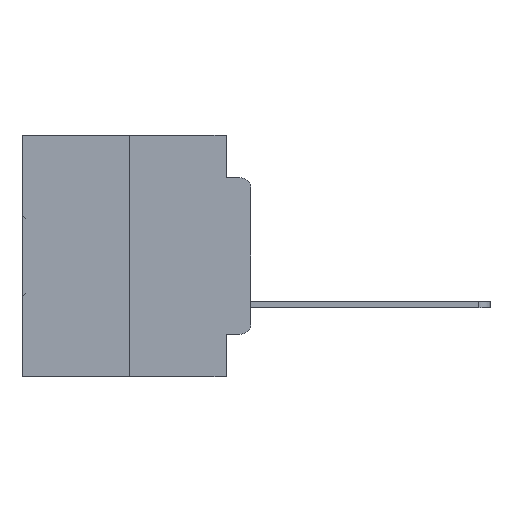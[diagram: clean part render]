
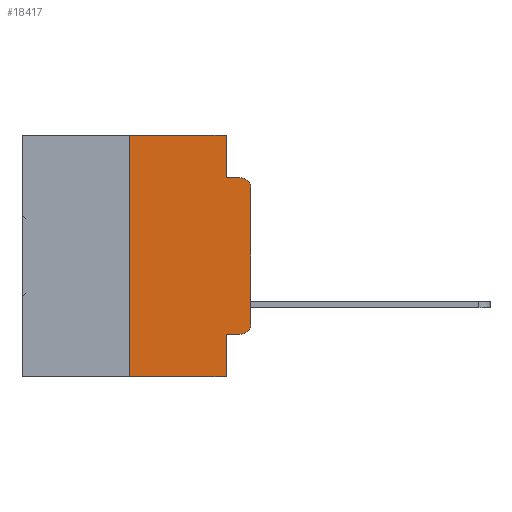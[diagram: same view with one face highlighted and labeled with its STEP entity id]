
A CAD part, left-side view. The second image highlights one B-rep face of the part: STEP entity #18417.
In plain terms, the highlighted planar face has unit normal (-1, 0, 0).
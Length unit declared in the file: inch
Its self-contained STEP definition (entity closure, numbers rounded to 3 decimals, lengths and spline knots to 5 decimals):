
#1 = LINE ( 'NONE', #24178, #26257 ) ;
#377 = VERTEX_POINT ( 'NONE', #13164 ) ;
#1495 = VECTOR ( 'NONE', #8526, 39.37008 ) ;
#1611 = DIRECTION ( 'NONE',  ( 0., -1., 0. ) ) ;
#2806 = DIRECTION ( 'NONE',  ( 0., 0., 1. ) ) ;
#3068 = CARTESIAN_POINT ( 'NONE',  ( 0., 0.051, -0.5 ) ) ;
#4232 = VERTEX_POINT ( 'NONE', #7900 ) ;
#4436 = LINE ( 'NONE', #25506, #17606 ) ;
#4638 = DIRECTION ( 'NONE',  ( -1., 0., 0. ) ) ;
#5345 = CARTESIAN_POINT ( 'NONE',  ( 0., 0.02, -0.4115 ) ) ;
#5774 = CARTESIAN_POINT ( 'NONE',  ( 0., 0.051, -0.0885 ) ) ;
#5888 = CARTESIAN_POINT ( 'NONE',  ( 0., 0.051, 0. ) ) ;
#7290 = LINE ( 'NONE', #23462, #27106 ) ;
#7723 = CARTESIAN_POINT ( 'NONE',  ( 0., 0.473, 0. ) ) ;
#7900 = CARTESIAN_POINT ( 'NONE',  ( 0., 0.051, -0.4115 ) ) ;
#8096 = CARTESIAN_POINT ( 'NONE',  ( 0., 0.25, -0.5 ) ) ;
#8526 = DIRECTION ( 'NONE',  ( 0., 0., -1. ) ) ;
#8541 = VECTOR ( 'NONE', #29583, 39.37008 ) ;
#10542 = AXIS2_PLACEMENT_3D ( 'NONE', #7723, #10728, #28582 ) ;
#10728 = DIRECTION ( 'NONE',  ( 1., 0., 0. ) ) ;
#11220 = EDGE_CURVE ( 'NONE', #17238, #21538, #22645, .T. ) ;
#11301 = CARTESIAN_POINT ( 'NONE',  ( 0., 0.051, -0.4115 ) ) ;
#12679 = LINE ( 'NONE', #18549, #31714 ) ;
#13164 = CARTESIAN_POINT ( 'NONE',  ( 0., 0., -0.3915 ) ) ;
#13211 = CARTESIAN_POINT ( 'NONE',  ( 0., 0.02, -0.0885 ) ) ;
#13950 = DIRECTION ( 'NONE',  ( 0., -1., 0. ) ) ;
#14076 = VERTEX_POINT ( 'NONE', #27800 ) ;
#14179 = CARTESIAN_POINT ( 'NONE',  ( 0., 0.02, -0.3915 ) ) ;
#15052 = EDGE_CURVE ( 'NONE', #30312, #26683, #1, .T. ) ;
#15330 = AXIS2_PLACEMENT_3D ( 'NONE', #20431, #4638, #23036 ) ;
#15544 = VERTEX_POINT ( 'NONE', #5345 ) ;
#15669 = VECTOR ( 'NONE', #1611, 39.37008 ) ;
#16342 = EDGE_CURVE ( 'NONE', #377, #14076, #29641, .T. ) ;
#16435 = EDGE_CURVE ( 'NONE', #14076, #24211, #20089, .T. ) ;
#16441 = EDGE_CURVE ( 'NONE', #29751, #24211, #4436, .T. ) ;
#16532 = EDGE_CURVE ( 'NONE', #21538, #29751, #7290, .T. ) ;
#16572 = EDGE_CURVE ( 'NONE', #30312, #17238, #12679, .T. ) ;
#16673 = EDGE_CURVE ( 'NONE', #4232, #26683, #22517, .T. ) ;
#16718 = EDGE_CURVE ( 'NONE', #4232, #15544, #28196, .T. ) ;
#16768 = EDGE_CURVE ( 'NONE', #15544, #377, #20056, .T. ) ;
#16825 = DIRECTION ( 'NONE',  ( 0., 0., -1. ) ) ;
#17199 = CARTESIAN_POINT ( 'NONE',  ( 0., 0., 0. ) ) ;
#17238 = VERTEX_POINT ( 'NONE', #22961 ) ;
#17606 = VECTOR ( 'NONE', #27891, 39.37008 ) ;
#18417 = ADVANCED_FACE ( 'NONE', ( #18856 ), #18539, .F. ) ;
#18539 = PLANE ( 'NONE',  #10542 ) ;
#18549 = CARTESIAN_POINT ( 'NONE',  ( 0., 0.25, 0. ) ) ;
#18856 = FACE_OUTER_BOUND ( 'NONE', #19057, .T. ) ;
#19057 = EDGE_LOOP ( 'NONE', ( #20546, #21865, #22122, #22243, #22372, #22690, #22718, #22985, #23258, #30840 ) ) ;
#20054 = CARTESIAN_POINT ( 'NONE',  ( 0., 0.473, 0. ) ) ;
#20056 = CIRCLE ( 'NONE', #26711, 0.02 ) ;
#20089 = CIRCLE ( 'NONE', #15330, 0.02 ) ;
#20431 = CARTESIAN_POINT ( 'NONE',  ( 0., 0.02, -0.1085 ) ) ;
#20546 = ORIENTED_EDGE ( 'NONE', *, *, #16342, .T. ) ;
#20883 = VECTOR ( 'NONE', #13950, 39.37008 ) ;
#21538 = VERTEX_POINT ( 'NONE', #26733 ) ;
#21865 = ORIENTED_EDGE ( 'NONE', *, *, #16435, .T. ) ;
#22122 = ORIENTED_EDGE ( 'NONE', *, *, #16441, .F. ) ;
#22243 = ORIENTED_EDGE ( 'NONE', *, *, #16532, .F. ) ;
#22372 = ORIENTED_EDGE ( 'NONE', *, *, #11220, .F. ) ;
#22517 = LINE ( 'NONE', #5888, #1495 ) ;
#22645 = LINE ( 'NONE', #20054, #15669 ) ;
#22690 = ORIENTED_EDGE ( 'NONE', *, *, #16572, .F. ) ;
#22718 = ORIENTED_EDGE ( 'NONE', *, *, #15052, .T. ) ;
#22961 = CARTESIAN_POINT ( 'NONE',  ( 0., 0.25, 0. ) ) ;
#22985 = ORIENTED_EDGE ( 'NONE', *, *, #16673, .F. ) ;
#23036 = DIRECTION ( 'NONE',  ( 0., 0., -1. ) ) ;
#23258 = ORIENTED_EDGE ( 'NONE', *, *, #16718, .T. ) ;
#23462 = CARTESIAN_POINT ( 'NONE',  ( 0., 0.051, 0. ) ) ;
#24178 = CARTESIAN_POINT ( 'NONE',  ( 0., 0.473, -0.5 ) ) ;
#24211 = VERTEX_POINT ( 'NONE', #13211 ) ;
#25506 = CARTESIAN_POINT ( 'NONE',  ( 0., 0.051, -0.0885 ) ) ;
#26257 = VECTOR ( 'NONE', #26592, 39.37008 ) ;
#26592 = DIRECTION ( 'NONE',  ( 0., -1., 0. ) ) ;
#26683 = VERTEX_POINT ( 'NONE', #3068 ) ;
#26711 = AXIS2_PLACEMENT_3D ( 'NONE', #14179, #31517, #16825 ) ;
#26733 = CARTESIAN_POINT ( 'NONE',  ( 0., 0.051, 0. ) ) ;
#27106 = VECTOR ( 'NONE', #28185, 39.37008 ) ;
#27800 = CARTESIAN_POINT ( 'NONE',  ( 0., 0., -0.1085 ) ) ;
#27891 = DIRECTION ( 'NONE',  ( 0., -1., 0. ) ) ;
#28185 = DIRECTION ( 'NONE',  ( 0., 0., -1. ) ) ;
#28196 = LINE ( 'NONE', #11301, #20883 ) ;
#28582 = DIRECTION ( 'NONE',  ( 0., 0., -1. ) ) ;
#29583 = DIRECTION ( 'NONE',  ( 0., 0., 1. ) ) ;
#29641 = LINE ( 'NONE', #17199, #8541 ) ;
#29751 = VERTEX_POINT ( 'NONE', #5774 ) ;
#30312 = VERTEX_POINT ( 'NONE', #8096 ) ;
#30840 = ORIENTED_EDGE ( 'NONE', *, *, #16768, .T. ) ;
#31517 = DIRECTION ( 'NONE',  ( -1., 0., 0. ) ) ;
#31714 = VECTOR ( 'NONE', #2806, 39.37008 ) ;
